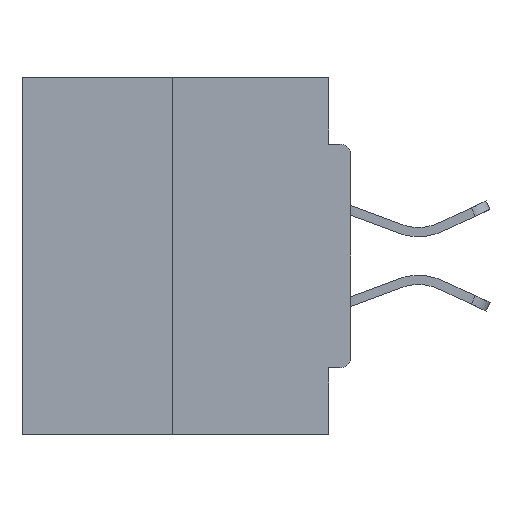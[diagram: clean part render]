
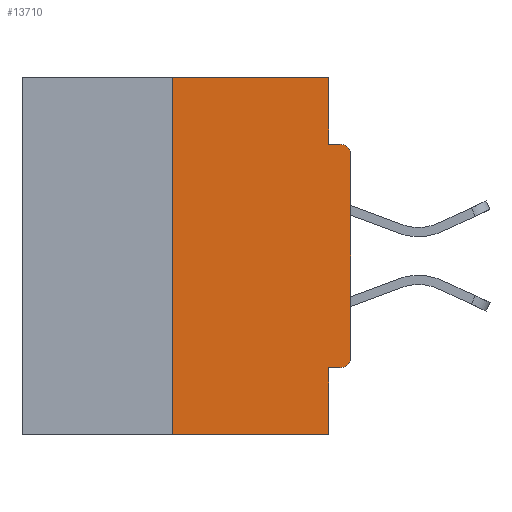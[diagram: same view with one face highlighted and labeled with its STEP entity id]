
A CAD part, left-side view. The second image highlights one B-rep face of the part: STEP entity #13710.
In plain terms, the highlighted planar face has unit normal (-1, 0, 0).
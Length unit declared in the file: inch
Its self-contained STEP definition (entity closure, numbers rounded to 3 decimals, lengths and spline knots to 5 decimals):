
#18 = VECTOR ( 'NONE', #16278, 39.37008 ) ;
#581 = VERTEX_POINT ( 'NONE', #8888 ) ;
#628 = EDGE_CURVE ( 'NONE', #14631, #27235, #30275, .T. ) ;
#846 = AXIS2_PLACEMENT_3D ( 'NONE', #21115, #13011, #18404 ) ;
#986 = LINE ( 'NONE', #11946, #31404 ) ;
#1205 = CARTESIAN_POINT ( 'NONE',  ( 0., 0.25, -0.5 ) ) ;
#1222 = CARTESIAN_POINT ( 'NONE',  ( 0., 0., 0. ) ) ;
#2051 = EDGE_CURVE ( 'NONE', #33614, #26737, #25665, .T. ) ;
#2453 = VERTEX_POINT ( 'NONE', #6013 ) ;
#2865 = ORIENTED_EDGE ( 'NONE', *, *, #4064, .F. ) ;
#3406 = VERTEX_POINT ( 'NONE', #1205 ) ;
#4064 = EDGE_CURVE ( 'NONE', #34940, #33614, #27559, .T. ) ;
#4693 = VECTOR ( 'NONE', #4908, 39.37008 ) ;
#4908 = DIRECTION ( 'NONE',  ( 0., -1., 0. ) ) ;
#5079 = CARTESIAN_POINT ( 'NONE',  ( 0., 0.46, -0.5 ) ) ;
#5136 = ORIENTED_EDGE ( 'NONE', *, *, #12623, .F. ) ;
#5165 = DIRECTION ( 'NONE',  ( 0., -1., 0. ) ) ;
#5883 = VECTOR ( 'NONE', #18143, 39.37008 ) ;
#6013 = CARTESIAN_POINT ( 'NONE',  ( 0., 0.031, -0.5 ) ) ;
#6873 = PLANE ( 'NONE',  #846 ) ;
#7162 = VECTOR ( 'NONE', #12902, 39.37008 ) ;
#7214 = DIRECTION ( 'NONE',  ( -1., 0., 0. ) ) ;
#7269 = CARTESIAN_POINT ( 'NONE',  ( 0., 0.015, -0.4065 ) ) ;
#7327 = LINE ( 'NONE', #13271, #7979 ) ;
#7958 = EDGE_CURVE ( 'NONE', #15929, #9136, #16099, .T. ) ;
#7979 = VECTOR ( 'NONE', #5165, 39.37008 ) ;
#8730 = VECTOR ( 'NONE', #24673, 39.37008 ) ;
#8888 = CARTESIAN_POINT ( 'NONE',  ( 0., 0., -0.3915 ) ) ;
#9136 = VERTEX_POINT ( 'NONE', #34697 ) ;
#9996 = LINE ( 'NONE', #26365, #18610 ) ;
#10122 = FACE_OUTER_BOUND ( 'NONE', #21147, .T. ) ;
#10162 = ORIENTED_EDGE ( 'NONE', *, *, #20315, .F. ) ;
#10355 = CARTESIAN_POINT ( 'NONE',  ( 0., 0.031, 0. ) ) ;
#11215 = CARTESIAN_POINT ( 'NONE',  ( 0., 0., -0.4065 ) ) ;
#11946 = CARTESIAN_POINT ( 'NONE',  ( 0., 0.031, -0.5 ) ) ;
#12623 = EDGE_CURVE ( 'NONE', #3406, #34940, #9996, .T. ) ;
#12824 = LINE ( 'NONE', #5079, #4693 ) ;
#12902 = DIRECTION ( 'NONE',  ( 0., 0., -1. ) ) ;
#13011 = DIRECTION ( 'NONE',  ( 1., 0., 0. ) ) ;
#13203 = CIRCLE ( 'NONE', #17205, 0.015 ) ;
#13271 = CARTESIAN_POINT ( 'NONE',  ( 0., 0., -0.0935 ) ) ;
#13710 = ADVANCED_FACE ( 'NONE', ( #10122 ), #6873, .F. ) ;
#13996 = ORIENTED_EDGE ( 'NONE', *, *, #15755, .F. ) ;
#14281 = CARTESIAN_POINT ( 'NONE',  ( 0., 0.015, -0.0935 ) ) ;
#14631 = VERTEX_POINT ( 'NONE', #29656 ) ;
#15585 = ORIENTED_EDGE ( 'NONE', *, *, #628, .T. ) ;
#15755 = EDGE_CURVE ( 'NONE', #9136, #2453, #986, .T. ) ;
#15929 = VERTEX_POINT ( 'NONE', #7269 ) ;
#16099 = LINE ( 'NONE', #11215, #18 ) ;
#16278 = DIRECTION ( 'NONE',  ( 0., 1., 0. ) ) ;
#16352 = CARTESIAN_POINT ( 'NONE',  ( 0., 0.031, -0.0935 ) ) ;
#16477 = DIRECTION ( 'NONE',  ( -1., 0., 0. ) ) ;
#16578 = CARTESIAN_POINT ( 'NONE',  ( 0., 0.46, 0. ) ) ;
#17098 = ORIENTED_EDGE ( 'NONE', *, *, #2051, .F. ) ;
#17205 = AXIS2_PLACEMENT_3D ( 'NONE', #23235, #7214, #28799 ) ;
#18143 = DIRECTION ( 'NONE',  ( 0., 0., 1. ) ) ;
#18404 = DIRECTION ( 'NONE',  ( 0., 0., -1. ) ) ;
#18610 = VECTOR ( 'NONE', #23679, 39.37008 ) ;
#18809 = AXIS2_PLACEMENT_3D ( 'NONE', #22571, #16477, #30846 ) ;
#20315 = EDGE_CURVE ( 'NONE', #26737, #27235, #7327, .T. ) ;
#21024 = ORIENTED_EDGE ( 'NONE', *, *, #7958, .F. ) ;
#21115 = CARTESIAN_POINT ( 'NONE',  ( 0., 0.46, 0. ) ) ;
#21147 = EDGE_LOOP ( 'NONE', ( #2865, #5136, #26115, #13996, #21024, #32803, #30707, #15585, #10162, #17098 ) ) ;
#22564 = EDGE_CURVE ( 'NONE', #15929, #581, #13203, .T. ) ;
#22571 = CARTESIAN_POINT ( 'NONE',  ( 0., 0.015, -0.1085 ) ) ;
#22926 = DIRECTION ( 'NONE',  ( 0., 0., -1. ) ) ;
#23235 = CARTESIAN_POINT ( 'NONE',  ( 0., 0.015, -0.3915 ) ) ;
#23679 = DIRECTION ( 'NONE',  ( 0., 0., 1. ) ) ;
#24673 = DIRECTION ( 'NONE',  ( 0., -1., 0. ) ) ;
#25665 = LINE ( 'NONE', #34137, #7162 ) ;
#25719 = CARTESIAN_POINT ( 'NONE',  ( 0., 0.25, 0. ) ) ;
#26115 = ORIENTED_EDGE ( 'NONE', *, *, #34509, .T. ) ;
#26365 = CARTESIAN_POINT ( 'NONE',  ( 0., 0.25, 0. ) ) ;
#26737 = VERTEX_POINT ( 'NONE', #16352 ) ;
#27235 = VERTEX_POINT ( 'NONE', #14281 ) ;
#27559 = LINE ( 'NONE', #16578, #8730 ) ;
#28799 = DIRECTION ( 'NONE',  ( 0., 0., -1. ) ) ;
#29656 = CARTESIAN_POINT ( 'NONE',  ( 0., 0., -0.1085 ) ) ;
#30275 = CIRCLE ( 'NONE', #18809, 0.015 ) ;
#30707 = ORIENTED_EDGE ( 'NONE', *, *, #35351, .T. ) ;
#30846 = DIRECTION ( 'NONE',  ( 0., 0., -1. ) ) ;
#31277 = LINE ( 'NONE', #1222, #5883 ) ;
#31404 = VECTOR ( 'NONE', #22926, 39.37008 ) ;
#32803 = ORIENTED_EDGE ( 'NONE', *, *, #22564, .T. ) ;
#33614 = VERTEX_POINT ( 'NONE', #10355 ) ;
#34137 = CARTESIAN_POINT ( 'NONE',  ( 0., 0.031, 0. ) ) ;
#34509 = EDGE_CURVE ( 'NONE', #3406, #2453, #12824, .T. ) ;
#34697 = CARTESIAN_POINT ( 'NONE',  ( 0., 0.031, -0.4065 ) ) ;
#34940 = VERTEX_POINT ( 'NONE', #25719 ) ;
#35351 = EDGE_CURVE ( 'NONE', #581, #14631, #31277, .T. ) ;
